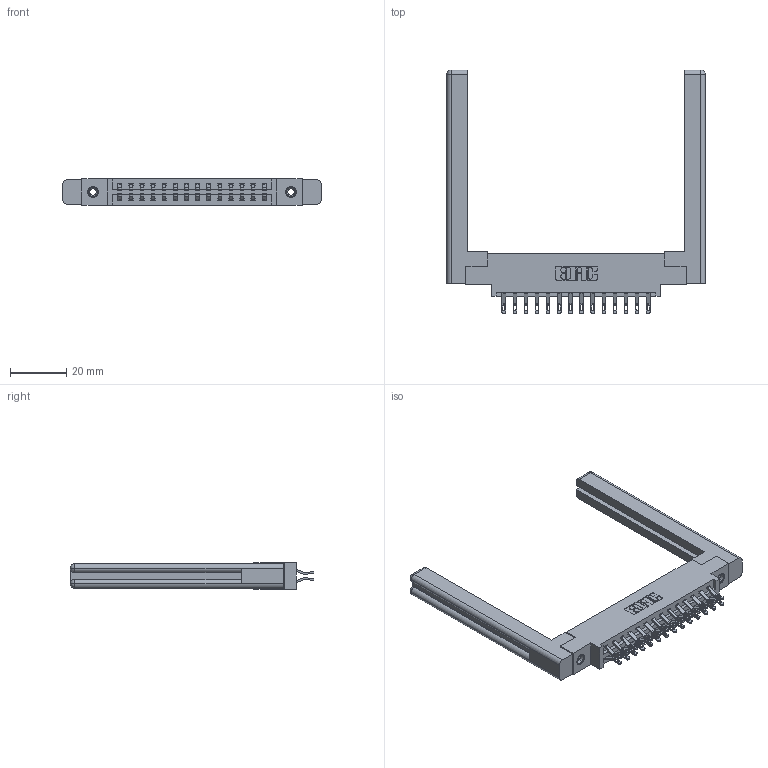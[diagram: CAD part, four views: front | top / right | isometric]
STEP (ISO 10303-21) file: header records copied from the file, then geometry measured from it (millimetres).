
FILE_DESCRIPTION (( 'STEP AP203' ), '1' );
FILE_NAME ('337-028-555-858.STEP', '2019-10-10T23:00:05', ( '' ), ( '' ), 'SwSTEP 2.0', 'SolidWorks 2016', '' );
FILE_SCHEMA (( 'CONFIG_CONTROL_DESIGN' ));
Length unit declared in the file: inch
Products named in the file (5): 337-028-555-858; 345-292-001_555 Tail; 337 Part_0.170 Offset - 0.156 Dia-TI; 345-250-001_345-250-001-102; 307-220-058
Assembly tree (33 placements, depth 2):
  337-028-555-858
    337 Part_0.170 Offset - 0.156 Dia-TI
    345-292-001_555 Tail  x28
    345-250-001_345-250-001-102  x2
    307-220-058  x2
Bounding box: 92.1 x 86.87 x 9.4 mm (x, y, z)
Volume: 16439.6 mm3; surface area: 15699.3 mm2
Topology: 33 solids, 33 shells, 1940 faces, 5969 edges, 3966 vertices
Faces by surface type: plane 1166, cylinder 750, cone 12, torus 12
Entity records: 17568 total; most frequent: CARTESIAN_POINT 3027, ORIENTED_EDGE 2872, DIRECTION 2612, EDGE_CURVE 1436, LINE 1240, VECTOR 1240, VERTEX_POINT 950, AXIS2_PLACEMENT_3D 686
